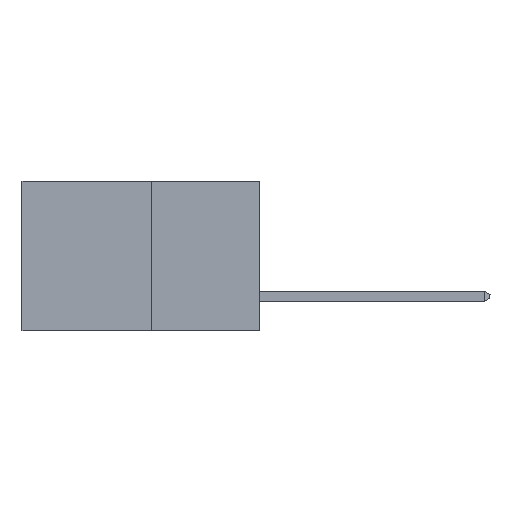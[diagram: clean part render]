
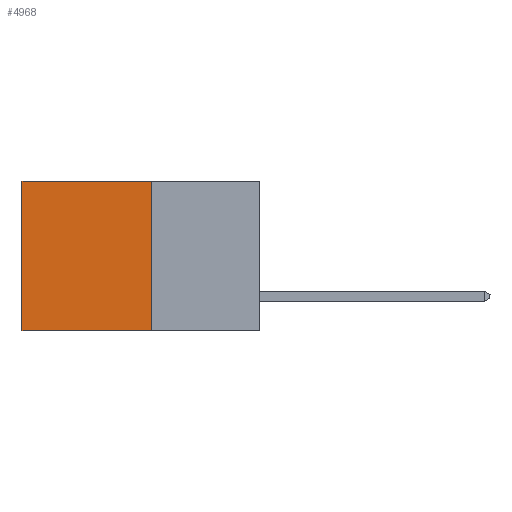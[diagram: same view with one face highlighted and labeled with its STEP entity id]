
A CAD part, left-side view. The second image highlights one B-rep face of the part: STEP entity #4968.
In plain terms, the highlighted planar face has unit normal (-1, 0, 0).
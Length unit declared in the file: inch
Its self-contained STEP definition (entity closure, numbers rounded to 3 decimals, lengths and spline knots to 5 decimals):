
#88 = EDGE_CURVE ( 'NONE', #2172, #4210, #8276, .T. ) ;
#212 = EDGE_LOOP ( 'NONE', ( #8702, #3896, #6002, #5011 ) ) ;
#531 = EDGE_CURVE ( 'NONE', #800, #4210, #2751, .T. ) ;
#800 = VERTEX_POINT ( 'NONE', #1578 ) ;
#1128 = CARTESIAN_POINT ( 'NONE',  ( 0.277, 0.59, 0. ) ) ;
#1133 = EDGE_CURVE ( 'NONE', #4627, #2172, #5212, .T. ) ;
#1578 = CARTESIAN_POINT ( 'NONE',  ( 0.277, 0.27, -0.37 ) ) ;
#1888 = CARTESIAN_POINT ( 'NONE',  ( 0.277, 0.27, -0.37 ) ) ;
#1948 = DIRECTION ( 'NONE',  ( 0., 0., -1. ) ) ;
#2172 = VERTEX_POINT ( 'NONE', #1128 ) ;
#2518 = VECTOR ( 'NONE', #4381, 39.37008 ) ;
#2644 = CARTESIAN_POINT ( 'NONE',  ( 0.277, 0.59, -0.37 ) ) ;
#2649 = DIRECTION ( 'NONE',  ( 0., 1., 0. ) ) ;
#2751 = LINE ( 'NONE', #4313, #8269 ) ;
#3769 = AXIS2_PLACEMENT_3D ( 'NONE', #7906, #8052, #8011 ) ;
#3896 = ORIENTED_EDGE ( 'NONE', *, *, #531, .F. ) ;
#4210 = VERTEX_POINT ( 'NONE', #2644 ) ;
#4313 = CARTESIAN_POINT ( 'NONE',  ( 0.277, 0.27, -0.37 ) ) ;
#4381 = DIRECTION ( 'NONE',  ( 0., 0., -1. ) ) ;
#4627 = VERTEX_POINT ( 'NONE', #9356 ) ;
#4769 = LINE ( 'NONE', #1888, #8337 ) ;
#4968 = ADVANCED_FACE ( 'NONE', ( #9301 ), #6587, .F. ) ;
#5011 = ORIENTED_EDGE ( 'NONE', *, *, #1133, .T. ) ;
#5212 = LINE ( 'NONE', #9018, #9030 ) ;
#6002 = ORIENTED_EDGE ( 'NONE', *, *, #7361, .F. ) ;
#6587 = PLANE ( 'NONE',  #3769 ) ;
#7361 = EDGE_CURVE ( 'NONE', #4627, #800, #4769, .T. ) ;
#7906 = CARTESIAN_POINT ( 'NONE',  ( 0.277, 0.27, -0.37 ) ) ;
#8011 = DIRECTION ( 'NONE',  ( 0., 0., -1. ) ) ;
#8052 = DIRECTION ( 'NONE',  ( 1., 0., 0. ) ) ;
#8269 = VECTOR ( 'NONE', #2649, 39.37008 ) ;
#8276 = LINE ( 'NONE', #8744, #2518 ) ;
#8337 = VECTOR ( 'NONE', #1948, 39.37008 ) ;
#8622 = DIRECTION ( 'NONE',  ( 0., 1., 0. ) ) ;
#8702 = ORIENTED_EDGE ( 'NONE', *, *, #88, .T. ) ;
#8744 = CARTESIAN_POINT ( 'NONE',  ( 0.277, 0.59, -0.37 ) ) ;
#9018 = CARTESIAN_POINT ( 'NONE',  ( 0.277, 0.27, 0. ) ) ;
#9030 = VECTOR ( 'NONE', #8622, 39.37008 ) ;
#9301 = FACE_OUTER_BOUND ( 'NONE', #212, .T. ) ;
#9356 = CARTESIAN_POINT ( 'NONE',  ( 0.277, 0.27, 0. ) ) ;
